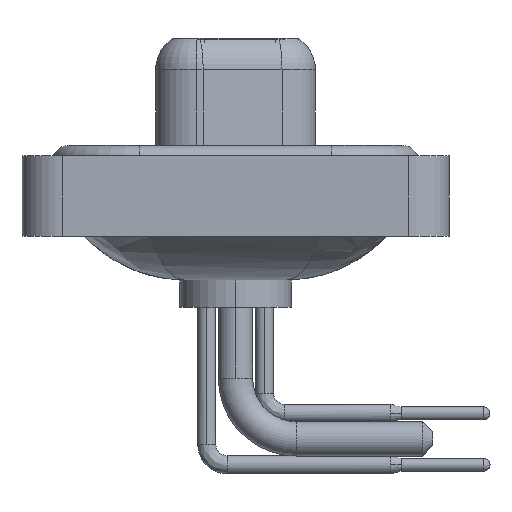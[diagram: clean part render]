
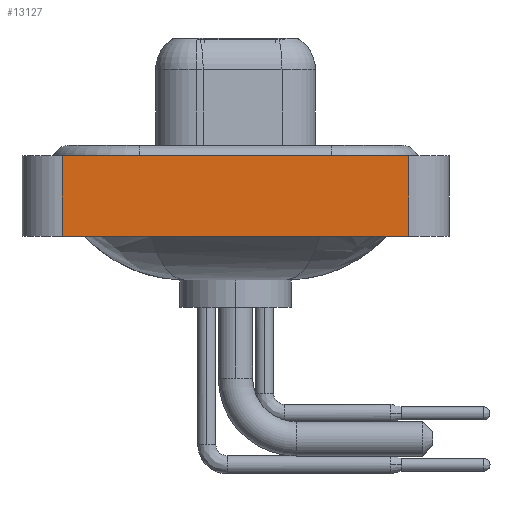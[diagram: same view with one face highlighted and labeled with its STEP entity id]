
A CAD part, left-side view. The second image highlights one B-rep face of the part: STEP entity #13127.
In plain terms, the highlighted planar face has unit normal (-1, 0, 0).
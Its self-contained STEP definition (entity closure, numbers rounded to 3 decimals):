
#582 = LINE ( 'NONE', #4238, #2764 ) ;
#751 = EDGE_CURVE ( 'NONE', #6708, #7814, #9002, .T. ) ;
#2588 = CARTESIAN_POINT ( 'NONE',  ( -7.35, -8.55, -3.6 ) ) ;
#2645 = LINE ( 'NONE', #9671, #21346 ) ;
#2654 = DIRECTION ( 'NONE',  ( -1., 0., 0. ) ) ;
#2719 = EDGE_LOOP ( 'NONE', ( #6597, #11589, #8361, #19806 ) ) ;
#2764 = VECTOR ( 'NONE', #18346, 1000. ) ;
#3805 = PLANE ( 'NONE',  #21755 ) ;
#4238 = CARTESIAN_POINT ( 'NONE',  ( -7.35, -8.55, 0.4 ) ) ;
#4285 = CARTESIAN_POINT ( 'NONE',  ( -7.35, 8.55, 0.4 ) ) ;
#4606 = CARTESIAN_POINT ( 'NONE',  ( -7.35, -8.55, 0.4 ) ) ;
#5255 = CARTESIAN_POINT ( 'NONE',  ( -7.35, 8.55, -3.6 ) ) ;
#6597 = ORIENTED_EDGE ( 'NONE', *, *, #15059, .T. ) ;
#6708 = VERTEX_POINT ( 'NONE', #5255 ) ;
#7814 = VERTEX_POINT ( 'NONE', #4285 ) ;
#8361 = ORIENTED_EDGE ( 'NONE', *, *, #751, .F. ) ;
#8395 = CARTESIAN_POINT ( 'NONE',  ( -7.35, -8.55, -3.6 ) ) ;
#9002 = LINE ( 'NONE', #16070, #15468 ) ;
#9671 = CARTESIAN_POINT ( 'NONE',  ( -7.35, -8.55, -3.6 ) ) ;
#10946 = DIRECTION ( 'NONE',  ( 0., 0., 1. ) ) ;
#11014 = EDGE_CURVE ( 'NONE', #7814, #11130, #582, .T. ) ;
#11130 = VERTEX_POINT ( 'NONE', #4606 ) ;
#11589 = ORIENTED_EDGE ( 'NONE', *, *, #11014, .F. ) ;
#13127 = ADVANCED_FACE ( 'NONE', ( #19655 ), #3805, .T. ) ;
#13824 = LINE ( 'NONE', #8395, #19482 ) ;
#15059 = EDGE_CURVE ( 'NONE', #16555, #11130, #2645, .T. ) ;
#15449 = DIRECTION ( 'NONE',  ( 0., -1., 0. ) ) ;
#15468 = VECTOR ( 'NONE', #10946, 1000. ) ;
#16070 = CARTESIAN_POINT ( 'NONE',  ( -7.35, 8.55, -3.6 ) ) ;
#16184 = CARTESIAN_POINT ( 'NONE',  ( -7.35, -8.55, -3.6 ) ) ;
#16508 = DIRECTION ( 'NONE',  ( 0., 0., 1. ) ) ;
#16555 = VERTEX_POINT ( 'NONE', #2588 ) ;
#17073 = EDGE_CURVE ( 'NONE', #6708, #16555, #13824, .T. ) ;
#18346 = DIRECTION ( 'NONE',  ( 0., -1., 0. ) ) ;
#19482 = VECTOR ( 'NONE', #15449, 1000. ) ;
#19655 = FACE_OUTER_BOUND ( 'NONE', #2719, .T. ) ;
#19806 = ORIENTED_EDGE ( 'NONE', *, *, #17073, .T. ) ;
#20889 = DIRECTION ( 'NONE',  ( 0., 0., 1. ) ) ;
#21346 = VECTOR ( 'NONE', #20889, 1000. ) ;
#21755 = AXIS2_PLACEMENT_3D ( 'NONE', #16184, #2654, #16508 ) ;
